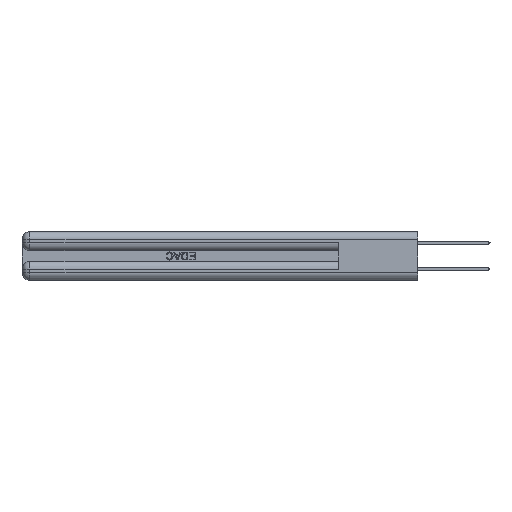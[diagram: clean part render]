
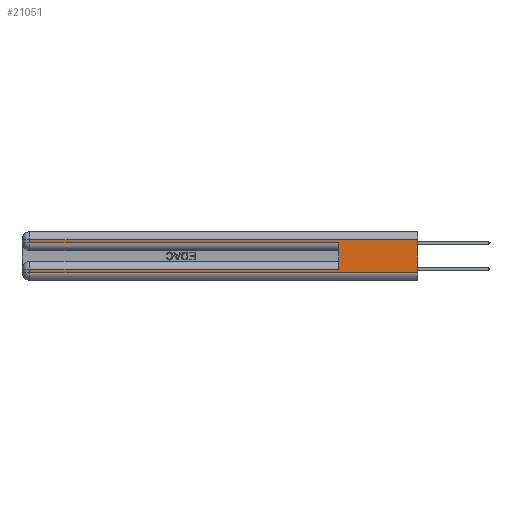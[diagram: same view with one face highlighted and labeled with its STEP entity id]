
A CAD part, left-side view. The second image highlights one B-rep face of the part: STEP entity #21051.
In plain terms, the highlighted planar face has unit normal (-1, 0, 0).
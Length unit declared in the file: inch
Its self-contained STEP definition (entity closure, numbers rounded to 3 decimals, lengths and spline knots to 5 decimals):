
#774 = VECTOR ( 'NONE', #990, 39.37008 ) ;
#990 = DIRECTION ( 'NONE',  ( 0., 0., -1. ) ) ;
#1159 = CARTESIAN_POINT ( 'NONE',  ( 0., 2.94, 0.06 ) ) ;
#1758 = VECTOR ( 'NONE', #10656, 39.37008 ) ;
#1919 = LINE ( 'NONE', #35270, #774 ) ;
#3691 = ORIENTED_EDGE ( 'NONE', *, *, #17899, .T. ) ;
#4008 = AXIS2_PLACEMENT_3D ( 'NONE', #32582, #21078, #34920 ) ;
#4801 = PLANE ( 'NONE',  #4008 ) ;
#4816 = VECTOR ( 'NONE', #35838, 39.37008 ) ;
#5909 = LINE ( 'NONE', #39452, #4816 ) ;
#6438 = DIRECTION ( 'NONE',  ( 0., 0., -1. ) ) ;
#6475 = ORIENTED_EDGE ( 'NONE', *, *, #23007, .F. ) ;
#7423 = LINE ( 'NONE', #15833, #12295 ) ;
#8183 = VERTEX_POINT ( 'NONE', #31856 ) ;
#8955 = EDGE_CURVE ( 'NONE', #41413, #37128, #1919, .T. ) ;
#9368 = ORIENTED_EDGE ( 'NONE', *, *, #12793, .T. ) ;
#9983 = DIRECTION ( 'NONE',  ( 0., 1., 0. ) ) ;
#10099 = VERTEX_POINT ( 'NONE', #1159 ) ;
#10656 = DIRECTION ( 'NONE',  ( 0., 0., -1. ) ) ;
#10702 = CARTESIAN_POINT ( 'NONE',  ( 0., 2.94, 0.085 ) ) ;
#12295 = VECTOR ( 'NONE', #6438, 39.37008 ) ;
#12380 = EDGE_CURVE ( 'NONE', #41413, #38902, #5909, .T. ) ;
#12434 = VECTOR ( 'NONE', #9983, 39.37008 ) ;
#12793 = EDGE_CURVE ( 'NONE', #10099, #37128, #33428, .T. ) ;
#14103 = CARTESIAN_POINT ( 'NONE',  ( 0., 0., 0.06 ) ) ;
#15833 = CARTESIAN_POINT ( 'NONE',  ( 0., 2.94, 0.37 ) ) ;
#16178 = LINE ( 'NONE', #36112, #24812 ) ;
#16381 = CARTESIAN_POINT ( 'NONE',  ( 0., 0., 0.085 ) ) ;
#17899 = EDGE_CURVE ( 'NONE', #8183, #23709, #16178, .T. ) ;
#18162 = ORIENTED_EDGE ( 'NONE', *, *, #35335, .T. ) ;
#19200 = FACE_OUTER_BOUND ( 'NONE', #28957, .T. ) ;
#19327 = EDGE_CURVE ( 'NONE', #41072, #10099, #7423, .T. ) ;
#19673 = CARTESIAN_POINT ( 'NONE',  ( 0., 0., 0.31 ) ) ;
#21051 = ADVANCED_FACE ( 'NONE', ( #19200 ), #4801, .F. ) ;
#21078 = DIRECTION ( 'NONE',  ( 1., 0., 0. ) ) ;
#21677 = LINE ( 'NONE', #16381, #12434 ) ;
#22934 = VECTOR ( 'NONE', #35755, 39.37008 ) ;
#23007 = EDGE_CURVE ( 'NONE', #32644, #23709, #29334, .T. ) ;
#23709 = VERTEX_POINT ( 'NONE', #25067 ) ;
#23964 = CARTESIAN_POINT ( 'NONE',  ( 0., 0., 0.06 ) ) ;
#24457 = CARTESIAN_POINT ( 'NONE',  ( 0., 2.94, 0.31 ) ) ;
#24812 = VECTOR ( 'NONE', #43042, 39.37008 ) ;
#25067 = CARTESIAN_POINT ( 'NONE',  ( 0., 0.6, 0.285 ) ) ;
#25581 = ORIENTED_EDGE ( 'NONE', *, *, #8955, .F. ) ;
#27855 = ORIENTED_EDGE ( 'NONE', *, *, #12380, .T. ) ;
#27914 = CARTESIAN_POINT ( 'NONE',  ( 0., 2.94, 0.37 ) ) ;
#28957 = EDGE_LOOP ( 'NONE', ( #25581, #27855, #18162, #3691, #6475, #32521, #43352, #9368 ) ) ;
#29334 = LINE ( 'NONE', #42543, #22934 ) ;
#31856 = CARTESIAN_POINT ( 'NONE',  ( 0., 2.94, 0.285 ) ) ;
#32521 = ORIENTED_EDGE ( 'NONE', *, *, #39005, .T. ) ;
#32582 = CARTESIAN_POINT ( 'NONE',  ( 0., 0., 0.37 ) ) ;
#32644 = VERTEX_POINT ( 'NONE', #41920 ) ;
#33388 = VECTOR ( 'NONE', #35501, 39.37008 ) ;
#33428 = LINE ( 'NONE', #23964, #33388 ) ;
#34920 = DIRECTION ( 'NONE',  ( 0., 0., -1. ) ) ;
#35270 = CARTESIAN_POINT ( 'NONE',  ( 0., 0., 0.37 ) ) ;
#35335 = EDGE_CURVE ( 'NONE', #38902, #8183, #44387, .T. ) ;
#35501 = DIRECTION ( 'NONE',  ( 0., -1., 0. ) ) ;
#35755 = DIRECTION ( 'NONE',  ( 0., 0., 1. ) ) ;
#35838 = DIRECTION ( 'NONE',  ( 0., 1., 0. ) ) ;
#36112 = CARTESIAN_POINT ( 'NONE',  ( 0., 0., 0.285 ) ) ;
#37128 = VERTEX_POINT ( 'NONE', #14103 ) ;
#38902 = VERTEX_POINT ( 'NONE', #24457 ) ;
#39005 = EDGE_CURVE ( 'NONE', #32644, #41072, #21677, .T. ) ;
#39452 = CARTESIAN_POINT ( 'NONE',  ( 0., 0., 0.31 ) ) ;
#41072 = VERTEX_POINT ( 'NONE', #10702 ) ;
#41413 = VERTEX_POINT ( 'NONE', #19673 ) ;
#41920 = CARTESIAN_POINT ( 'NONE',  ( 0., 0.6, 0.085 ) ) ;
#42543 = CARTESIAN_POINT ( 'NONE',  ( 0., 0.6, 0.145 ) ) ;
#43042 = DIRECTION ( 'NONE',  ( 0., -1., 0. ) ) ;
#43352 = ORIENTED_EDGE ( 'NONE', *, *, #19327, .T. ) ;
#44387 = LINE ( 'NONE', #27914, #1758 ) ;
